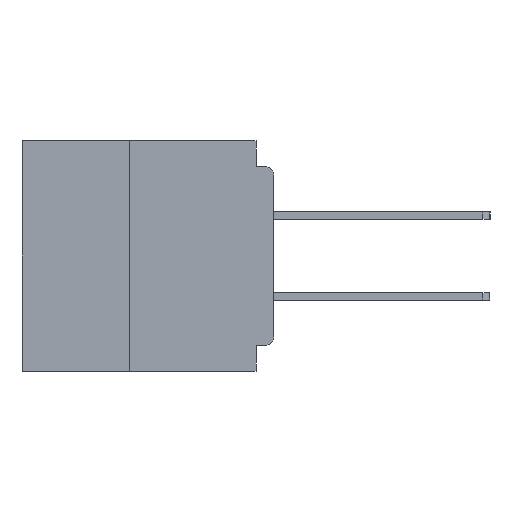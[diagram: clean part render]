
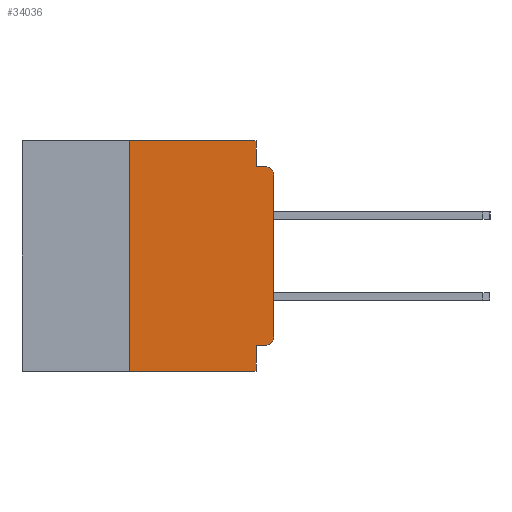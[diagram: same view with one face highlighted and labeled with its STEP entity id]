
A CAD part, left-side view. The second image highlights one B-rep face of the part: STEP entity #34036.
In plain terms, the highlighted planar face has unit normal (-1, 0, 0).
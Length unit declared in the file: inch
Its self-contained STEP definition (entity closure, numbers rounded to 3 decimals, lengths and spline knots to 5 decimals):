
#126 = ORIENTED_EDGE ( 'NONE', *, *, #11168, .F. ) ;
#341 = CIRCLE ( 'NONE', #40922, 0.015 ) ;
#1475 = CARTESIAN_POINT ( 'NONE',  ( 0., 0.031, -0.355 ) ) ;
#1499 = LINE ( 'NONE', #13170, #38092 ) ;
#1831 = AXIS2_PLACEMENT_3D ( 'NONE', #40200, #11657, #44871 ) ;
#2039 = CARTESIAN_POINT ( 'NONE',  ( 0., 0., -0.355 ) ) ;
#3531 = DIRECTION ( 'NONE',  ( 0., -1., 0. ) ) ;
#3682 = CARTESIAN_POINT ( 'NONE',  ( 0., 0., -0.06 ) ) ;
#3732 = VECTOR ( 'NONE', #53752, 39.37008 ) ;
#4075 = VERTEX_POINT ( 'NONE', #25786 ) ;
#5099 = VERTEX_POINT ( 'NONE', #29960 ) ;
#5710 = CARTESIAN_POINT ( 'NONE',  ( 0., 0.031, 0. ) ) ;
#5877 = VERTEX_POINT ( 'NONE', #49181 ) ;
#6510 = LINE ( 'NONE', #8980, #30486 ) ;
#7304 = VERTEX_POINT ( 'NONE', #60023 ) ;
#7401 = ORIENTED_EDGE ( 'NONE', *, *, #11288, .F. ) ;
#8049 = CARTESIAN_POINT ( 'NONE',  ( 0., 0.031, 0. ) ) ;
#8325 = VECTOR ( 'NONE', #31897, 39.37008 ) ;
#8708 = CARTESIAN_POINT ( 'NONE',  ( 0., 0.437, -0.4 ) ) ;
#8980 = CARTESIAN_POINT ( 'NONE',  ( 0., 0.031, -0.4 ) ) ;
#9238 = VECTOR ( 'NONE', #58989, 39.37008 ) ;
#9834 = LINE ( 'NONE', #8049, #8325 ) ;
#10637 = FACE_OUTER_BOUND ( 'NONE', #12742, .T. ) ;
#11168 = EDGE_CURVE ( 'NONE', #5877, #48375, #26780, .T. ) ;
#11288 = EDGE_CURVE ( 'NONE', #15384, #7304, #6510, .T. ) ;
#11559 = ORIENTED_EDGE ( 'NONE', *, *, #45294, .T. ) ;
#11657 = DIRECTION ( 'NONE',  ( 1., 0., 0. ) ) ;
#12742 = EDGE_LOOP ( 'NONE', ( #18926, #56367, #126, #44793, #27808, #37275, #11559, #7401, #16619, #51933 ) ) ;
#13170 = CARTESIAN_POINT ( 'NONE',  ( 0., 0.437, 0. ) ) ;
#13809 = CARTESIAN_POINT ( 'NONE',  ( 0., 0.25, 0. ) ) ;
#14054 = VECTOR ( 'NONE', #32039, 39.37008 ) ;
#14184 = EDGE_CURVE ( 'NONE', #4075, #15384, #33196, .T. ) ;
#15384 = VERTEX_POINT ( 'NONE', #1475 ) ;
#16544 = LINE ( 'NONE', #20680, #3732 ) ;
#16619 = ORIENTED_EDGE ( 'NONE', *, *, #14184, .F. ) ;
#16935 = EDGE_CURVE ( 'NONE', #49580, #30296, #16544, .T. ) ;
#18926 = ORIENTED_EDGE ( 'NONE', *, *, #61571, .T. ) ;
#18960 = CARTESIAN_POINT ( 'NONE',  ( 0., 0.015, -0.06 ) ) ;
#19190 = CARTESIAN_POINT ( 'NONE',  ( 0., 0.015, -0.34 ) ) ;
#19333 = AXIS2_PLACEMENT_3D ( 'NONE', #18960, #52025, #23764 ) ;
#20228 = LINE ( 'NONE', #8708, #56470 ) ;
#20680 = CARTESIAN_POINT ( 'NONE',  ( 0., 0.25, -0.4 ) ) ;
#23764 = DIRECTION ( 'NONE',  ( 0., 0., -1. ) ) ;
#23980 = DIRECTION ( 'NONE',  ( 0., 0., -1. ) ) ;
#25764 = VERTEX_POINT ( 'NONE', #3682 ) ;
#25786 = CARTESIAN_POINT ( 'NONE',  ( 0., 0.015, -0.355 ) ) ;
#26780 = LINE ( 'NONE', #27226, #14054 ) ;
#27192 = DIRECTION ( 'NONE',  ( 0., 0., 1. ) ) ;
#27226 = CARTESIAN_POINT ( 'NONE',  ( 0., 0., -0.045 ) ) ;
#27808 = ORIENTED_EDGE ( 'NONE', *, *, #50345, .F. ) ;
#29899 = VECTOR ( 'NONE', #27192, 39.37008 ) ;
#29960 = CARTESIAN_POINT ( 'NONE',  ( 0., 0., -0.34 ) ) ;
#30296 = VERTEX_POINT ( 'NONE', #13809 ) ;
#30486 = VECTOR ( 'NONE', #46986, 39.37008 ) ;
#31897 = DIRECTION ( 'NONE',  ( 0., 0., -1. ) ) ;
#32039 = DIRECTION ( 'NONE',  ( 0., -1., 0. ) ) ;
#32442 = EDGE_CURVE ( 'NONE', #4075, #5099, #341, .T. ) ;
#33196 = LINE ( 'NONE', #2039, #9238 ) ;
#34036 = ADVANCED_FACE ( 'NONE', ( #10637 ), #49387, .F. ) ;
#37275 = ORIENTED_EDGE ( 'NONE', *, *, #16935, .F. ) ;
#38092 = VECTOR ( 'NONE', #3531, 39.37008 ) ;
#40200 = CARTESIAN_POINT ( 'NONE',  ( 0., 0.437, 0. ) ) ;
#40448 = CARTESIAN_POINT ( 'NONE',  ( 0., 0.015, -0.045 ) ) ;
#40922 = AXIS2_PLACEMENT_3D ( 'NONE', #19190, #52250, #23980 ) ;
#42430 = LINE ( 'NONE', #46133, #29899 ) ;
#43493 = EDGE_CURVE ( 'NONE', #25764, #48375, #56571, .T. ) ;
#44793 = ORIENTED_EDGE ( 'NONE', *, *, #60349, .F. ) ;
#44871 = DIRECTION ( 'NONE',  ( 0., 0., -1. ) ) ;
#45294 = EDGE_CURVE ( 'NONE', #49580, #7304, #20228, .T. ) ;
#46133 = CARTESIAN_POINT ( 'NONE',  ( 0., 0., 0. ) ) ;
#46986 = DIRECTION ( 'NONE',  ( 0., 0., -1. ) ) ;
#48375 = VERTEX_POINT ( 'NONE', #40448 ) ;
#49181 = CARTESIAN_POINT ( 'NONE',  ( 0., 0.031, -0.045 ) ) ;
#49387 = PLANE ( 'NONE',  #1831 ) ;
#49580 = VERTEX_POINT ( 'NONE', #55150 ) ;
#50345 = EDGE_CURVE ( 'NONE', #30296, #54015, #1499, .T. ) ;
#51933 = ORIENTED_EDGE ( 'NONE', *, *, #32442, .T. ) ;
#52025 = DIRECTION ( 'NONE',  ( -1., 0., 0. ) ) ;
#52250 = DIRECTION ( 'NONE',  ( -1., 0., 0. ) ) ;
#53752 = DIRECTION ( 'NONE',  ( 0., 0., 1. ) ) ;
#54015 = VERTEX_POINT ( 'NONE', #5710 ) ;
#55150 = CARTESIAN_POINT ( 'NONE',  ( 0., 0.25, -0.4 ) ) ;
#56367 = ORIENTED_EDGE ( 'NONE', *, *, #43493, .T. ) ;
#56470 = VECTOR ( 'NONE', #61009, 39.37008 ) ;
#56571 = CIRCLE ( 'NONE', #19333, 0.015 ) ;
#58989 = DIRECTION ( 'NONE',  ( 0., 1., 0. ) ) ;
#60023 = CARTESIAN_POINT ( 'NONE',  ( 0., 0.031, -0.4 ) ) ;
#60349 = EDGE_CURVE ( 'NONE', #54015, #5877, #9834, .T. ) ;
#61009 = DIRECTION ( 'NONE',  ( 0., -1., 0. ) ) ;
#61571 = EDGE_CURVE ( 'NONE', #5099, #25764, #42430, .T. ) ;
